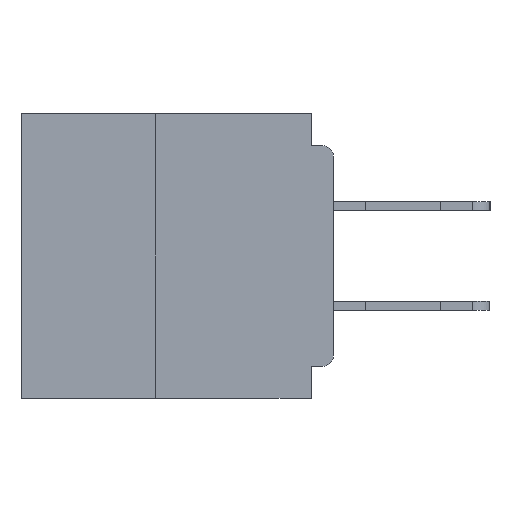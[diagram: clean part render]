
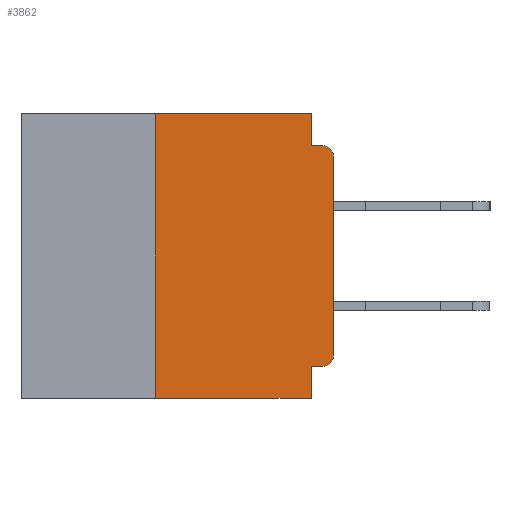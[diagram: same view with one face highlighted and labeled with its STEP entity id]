
A CAD part, left-side view. The second image highlights one B-rep face of the part: STEP entity #3862.
In plain terms, the highlighted planar face has unit normal (-1, 0, 0).
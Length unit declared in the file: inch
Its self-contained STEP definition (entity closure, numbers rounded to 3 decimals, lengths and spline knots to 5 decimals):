
#355 = DIRECTION ( 'NONE',  ( 0., 0., -1. ) ) ;
#642 = VECTOR ( 'NONE', #37462, 39.37008 ) ;
#1743 = LINE ( 'NONE', #19481, #25868 ) ;
#1886 = CARTESIAN_POINT ( 'NONE',  ( 0., 0., -0.045 ) ) ;
#1899 = VECTOR ( 'NONE', #21961, 39.37008 ) ;
#1973 = VERTEX_POINT ( 'NONE', #27557 ) ;
#3205 = ORIENTED_EDGE ( 'NONE', *, *, #30936, .T. ) ;
#3862 = ADVANCED_FACE ( 'NONE', ( #35769 ), #24427, .F. ) ;
#4845 = DIRECTION ( 'NONE',  ( 1., 0., 0. ) ) ;
#5266 = CARTESIAN_POINT ( 'NONE',  ( 0., 0.25, -0.4 ) ) ;
#5267 = DIRECTION ( 'NONE',  ( 0., -1., 0. ) ) ;
#5662 = CARTESIAN_POINT ( 'NONE',  ( 0., 0., 0. ) ) ;
#6331 = CARTESIAN_POINT ( 'NONE',  ( 0., 0., -0.06 ) ) ;
#6529 = LINE ( 'NONE', #14984, #7578 ) ;
#6903 = VECTOR ( 'NONE', #355, 39.37008 ) ;
#7013 = ORIENTED_EDGE ( 'NONE', *, *, #12621, .T. ) ;
#7578 = VECTOR ( 'NONE', #18252, 39.37008 ) ;
#8572 = CIRCLE ( 'NONE', #30283, 0.015 ) ;
#8683 = CARTESIAN_POINT ( 'NONE',  ( 0., 0.437, 0. ) ) ;
#9015 = CARTESIAN_POINT ( 'NONE',  ( 0., 0.031, -0.355 ) ) ;
#9178 = EDGE_LOOP ( 'NONE', ( #3205, #7013, #35338, #19041, #17547, #38884, #24868, #27074, #33638, #24594 ) ) ;
#9934 = CARTESIAN_POINT ( 'NONE',  ( 0., 0.015, -0.06 ) ) ;
#10033 = CARTESIAN_POINT ( 'NONE',  ( 0., 0.031, -0.045 ) ) ;
#10227 = CARTESIAN_POINT ( 'NONE',  ( 0., 0.031, 0. ) ) ;
#10370 = CIRCLE ( 'NONE', #39123, 0.015 ) ;
#11979 = DIRECTION ( 'NONE',  ( 0., -1., 0. ) ) ;
#12488 = EDGE_CURVE ( 'NONE', #17055, #28034, #12679, .T. ) ;
#12621 = EDGE_CURVE ( 'NONE', #31575, #23853, #8572, .T. ) ;
#12674 = DIRECTION ( 'NONE',  ( -1., 0., 0. ) ) ;
#12679 = LINE ( 'NONE', #32047, #21340 ) ;
#13225 = DIRECTION ( 'NONE',  ( 0., 0., -1. ) ) ;
#14536 = VERTEX_POINT ( 'NONE', #30820 ) ;
#14984 = CARTESIAN_POINT ( 'NONE',  ( 0., 0., -0.355 ) ) ;
#15017 = LINE ( 'NONE', #10227, #6903 ) ;
#16701 = LINE ( 'NONE', #1886, #41609 ) ;
#17055 = VERTEX_POINT ( 'NONE', #5266 ) ;
#17547 = ORIENTED_EDGE ( 'NONE', *, *, #35884, .F. ) ;
#18170 = LINE ( 'NONE', #21125, #642 ) ;
#18252 = DIRECTION ( 'NONE',  ( 0., 1., 0. ) ) ;
#18492 = VERTEX_POINT ( 'NONE', #10033 ) ;
#19041 = ORIENTED_EDGE ( 'NONE', *, *, #35163, .F. ) ;
#19481 = CARTESIAN_POINT ( 'NONE',  ( 0., 0.25, -0.4 ) ) ;
#19604 = VECTOR ( 'NONE', #11979, 39.37008 ) ;
#19639 = EDGE_CURVE ( 'NONE', #32366, #14536, #10370, .T. ) ;
#20188 = CARTESIAN_POINT ( 'NONE',  ( 0., 0.25, 0. ) ) ;
#21001 = CARTESIAN_POINT ( 'NONE',  ( 0., 0.437, 0. ) ) ;
#21125 = CARTESIAN_POINT ( 'NONE',  ( 0., 0.031, -0.4 ) ) ;
#21340 = VECTOR ( 'NONE', #38542, 39.37008 ) ;
#21420 = LINE ( 'NONE', #5662, #1899 ) ;
#21961 = DIRECTION ( 'NONE',  ( 0., 0., 1. ) ) ;
#22858 = EDGE_CURVE ( 'NONE', #41503, #28034, #18170, .T. ) ;
#22916 = EDGE_CURVE ( 'NONE', #18492, #23853, #16701, .T. ) ;
#23853 = VERTEX_POINT ( 'NONE', #35947 ) ;
#24427 = PLANE ( 'NONE',  #41326 ) ;
#24594 = ORIENTED_EDGE ( 'NONE', *, *, #19639, .T. ) ;
#24868 = ORIENTED_EDGE ( 'NONE', *, *, #12488, .T. ) ;
#25868 = VECTOR ( 'NONE', #35801, 39.37008 ) ;
#26631 = VERTEX_POINT ( 'NONE', #20188 ) ;
#27074 = ORIENTED_EDGE ( 'NONE', *, *, #22858, .F. ) ;
#27557 = CARTESIAN_POINT ( 'NONE',  ( 0., 0.031, 0. ) ) ;
#27717 = DIRECTION ( 'NONE',  ( 0., 0., -1. ) ) ;
#28034 = VERTEX_POINT ( 'NONE', #36420 ) ;
#28302 = LINE ( 'NONE', #8683, #19604 ) ;
#30283 = AXIS2_PLACEMENT_3D ( 'NONE', #9934, #32723, #13225 ) ;
#30820 = CARTESIAN_POINT ( 'NONE',  ( 0., 0., -0.34 ) ) ;
#30936 = EDGE_CURVE ( 'NONE', #14536, #31575, #21420, .T. ) ;
#31575 = VERTEX_POINT ( 'NONE', #6331 ) ;
#32047 = CARTESIAN_POINT ( 'NONE',  ( 0., 0.437, -0.4 ) ) ;
#32193 = CARTESIAN_POINT ( 'NONE',  ( 0., 0.015, -0.34 ) ) ;
#32366 = VERTEX_POINT ( 'NONE', #36314 ) ;
#32723 = DIRECTION ( 'NONE',  ( -1., 0., 0. ) ) ;
#33638 = ORIENTED_EDGE ( 'NONE', *, *, #40131, .F. ) ;
#33795 = EDGE_CURVE ( 'NONE', #17055, #26631, #1743, .T. ) ;
#35163 = EDGE_CURVE ( 'NONE', #1973, #18492, #15017, .T. ) ;
#35338 = ORIENTED_EDGE ( 'NONE', *, *, #22916, .F. ) ;
#35409 = DIRECTION ( 'NONE',  ( 0., 0., -1. ) ) ;
#35769 = FACE_OUTER_BOUND ( 'NONE', #9178, .T. ) ;
#35801 = DIRECTION ( 'NONE',  ( 0., 0., 1. ) ) ;
#35884 = EDGE_CURVE ( 'NONE', #26631, #1973, #28302, .T. ) ;
#35947 = CARTESIAN_POINT ( 'NONE',  ( 0., 0.015, -0.045 ) ) ;
#36314 = CARTESIAN_POINT ( 'NONE',  ( 0., 0.015, -0.355 ) ) ;
#36420 = CARTESIAN_POINT ( 'NONE',  ( 0., 0.031, -0.4 ) ) ;
#37462 = DIRECTION ( 'NONE',  ( 0., 0., -1. ) ) ;
#38542 = DIRECTION ( 'NONE',  ( 0., -1., 0. ) ) ;
#38884 = ORIENTED_EDGE ( 'NONE', *, *, #33795, .F. ) ;
#39123 = AXIS2_PLACEMENT_3D ( 'NONE', #32193, #12674, #35409 ) ;
#40131 = EDGE_CURVE ( 'NONE', #32366, #41503, #6529, .T. ) ;
#41326 = AXIS2_PLACEMENT_3D ( 'NONE', #21001, #4845, #27717 ) ;
#41503 = VERTEX_POINT ( 'NONE', #9015 ) ;
#41609 = VECTOR ( 'NONE', #5267, 39.37008 ) ;
